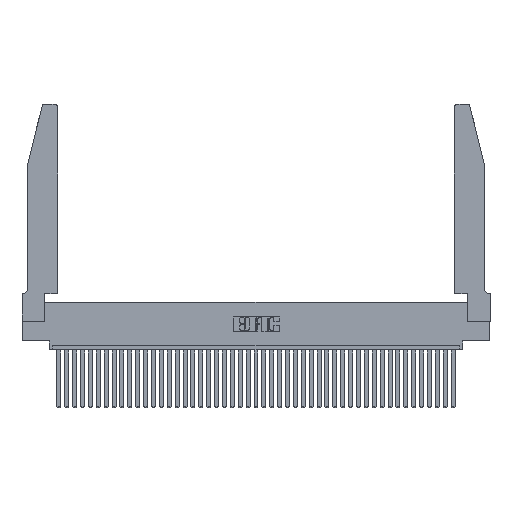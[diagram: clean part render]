
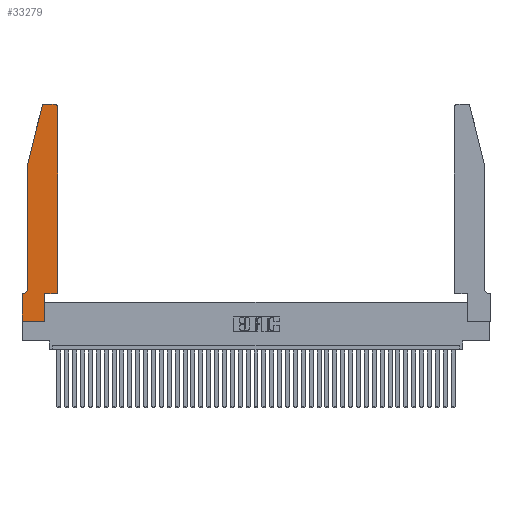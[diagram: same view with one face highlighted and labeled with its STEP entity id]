
A CAD part, top view. The second image highlights one B-rep face of the part: STEP entity #33279.
In plain terms, the highlighted planar face has unit normal (0, 0, 1).
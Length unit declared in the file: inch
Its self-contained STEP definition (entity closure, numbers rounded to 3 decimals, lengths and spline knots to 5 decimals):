
#1455 = CARTESIAN_POINT ( 'NONE',  ( 0., 0., 0.37 ) ) ;
#1532 = VECTOR ( 'NONE', #4703, 39.37008 ) ;
#1600 = DIRECTION ( 'NONE',  ( 0., 0., 1. ) ) ;
#2102 = EDGE_LOOP ( 'NONE', ( #39607, #27556, #12529, #35058, #14819, #30867, #3938, #31750, #32118, #39137, #9806, #36656 ) ) ;
#2121 = VERTEX_POINT ( 'NONE', #36961 ) ;
#2141 = CARTESIAN_POINT ( 'NONE',  ( 0.4205, 2.75, 0.37 ) ) ;
#2485 = VERTEX_POINT ( 'NONE', #36831 ) ;
#3154 = LINE ( 'NONE', #30062, #37539 ) ;
#3652 = CARTESIAN_POINT ( 'NONE',  ( 0., 0.35, 0.37 ) ) ;
#3937 = CIRCLE ( 'NONE', #37982, 0.03 ) ;
#3938 = ORIENTED_EDGE ( 'NONE', *, *, #39752, .T. ) ;
#4184 = LINE ( 'NONE', #41840, #13765 ) ;
#4213 = EDGE_CURVE ( 'NONE', #27043, #18013, #21855, .T. ) ;
#4671 = EDGE_CURVE ( 'NONE', #18013, #10865, #3154, .T. ) ;
#4703 = DIRECTION ( 'NONE',  ( 0., -1., 0. ) ) ;
#4770 = DIRECTION ( 'NONE',  ( 0., -1., 0. ) ) ;
#5153 = VERTEX_POINT ( 'NONE', #20958 ) ;
#6233 = VERTEX_POINT ( 'NONE', #3652 ) ;
#6235 = VECTOR ( 'NONE', #11917, 39.37008 ) ;
#6314 = CARTESIAN_POINT ( 'NONE',  ( 0.0755, 0.35, 0.37 ) ) ;
#7148 = EDGE_CURVE ( 'NONE', #34608, #27043, #18597, .T. ) ;
#7375 = VECTOR ( 'NONE', #31268, 39.37008 ) ;
#8874 = VECTOR ( 'NONE', #19285, 39.37008 ) ;
#8902 = EDGE_CURVE ( 'NONE', #31898, #6233, #24547, .T. ) ;
#9806 = ORIENTED_EDGE ( 'NONE', *, *, #24283, .T. ) ;
#10533 = EDGE_CURVE ( 'NONE', #2485, #30941, #40522, .T. ) ;
#10865 = VERTEX_POINT ( 'NONE', #31707 ) ;
#11106 = CARTESIAN_POINT ( 'NONE',  ( 0.284, 2.75, 0.37 ) ) ;
#11202 = DIRECTION ( 'NONE',  ( 1., 0., 0. ) ) ;
#11733 = CARTESIAN_POINT ( 'NONE',  ( 0.0055, 0.42, 0.37 ) ) ;
#11917 = DIRECTION ( 'NONE',  ( -0.239, -0.971, 0. ) ) ;
#12143 = AXIS2_PLACEMENT_3D ( 'NONE', #37515, #18132, #11202 ) ;
#12529 = ORIENTED_EDGE ( 'NONE', *, *, #4213, .T. ) ;
#12607 = VERTEX_POINT ( 'NONE', #2141 ) ;
#13274 = CARTESIAN_POINT ( 'NONE',  ( 0.4505, 0.35, 0.37 ) ) ;
#13550 = LINE ( 'NONE', #20067, #39370 ) ;
#13765 = VECTOR ( 'NONE', #19507, 39.37008 ) ;
#14819 = ORIENTED_EDGE ( 'NONE', *, *, #23988, .T. ) ;
#15023 = DIRECTION ( 'NONE',  ( 0., 0., -1. ) ) ;
#18013 = VERTEX_POINT ( 'NONE', #35134 ) ;
#18132 = DIRECTION ( 'NONE',  ( 0., 0., 1. ) ) ;
#18597 = CIRCLE ( 'NONE', #27298, 0.03 ) ;
#19285 = DIRECTION ( 'NONE',  ( -1., 0., 0. ) ) ;
#19507 = DIRECTION ( 'NONE',  ( 0., 1., 0. ) ) ;
#19769 = DIRECTION ( 'NONE',  ( 0., 1., 0. ) ) ;
#20067 = CARTESIAN_POINT ( 'NONE',  ( 0.2605, 2.75, 0.37 ) ) ;
#20542 = EDGE_CURVE ( 'NONE', #2121, #2485, #38345, .T. ) ;
#20958 = CARTESIAN_POINT ( 'NONE',  ( 0.4505, 2.72, 0.37 ) ) ;
#21148 = DIRECTION ( 'NONE',  ( 0., 0., 1. ) ) ;
#21514 = DIRECTION ( 'NONE',  ( -1., 0., 0. ) ) ;
#21816 = CARTESIAN_POINT ( 'NONE',  ( 0.0755, 2., 0.37 ) ) ;
#21855 = LINE ( 'NONE', #21816, #6235 ) ;
#22780 = CARTESIAN_POINT ( 'NONE',  ( 0.2865, 0.35, 0.37 ) ) ;
#23559 = AXIS2_PLACEMENT_3D ( 'NONE', #11733, #15023, #21514 ) ;
#23988 = EDGE_CURVE ( 'NONE', #10865, #31898, #40103, .T. ) ;
#24283 = EDGE_CURVE ( 'NONE', #30941, #5153, #4184, .T. ) ;
#24480 = FACE_OUTER_BOUND ( 'NONE', #2102, .T. ) ;
#24547 = LINE ( 'NONE', #6314, #8874 ) ;
#24636 = CARTESIAN_POINT ( 'NONE',  ( 0., 0., 0.37 ) ) ;
#25281 = CARTESIAN_POINT ( 'NONE',  ( 0.4505, 0.35, 0.37 ) ) ;
#27026 = EDGE_CURVE ( 'NONE', #12607, #34608, #13550, .T. ) ;
#27043 = VERTEX_POINT ( 'NONE', #30550 ) ;
#27231 = VECTOR ( 'NONE', #19769, 39.37008 ) ;
#27298 = AXIS2_PLACEMENT_3D ( 'NONE', #40869, #1600, #37095 ) ;
#27556 = ORIENTED_EDGE ( 'NONE', *, *, #7148, .T. ) ;
#27663 = DIRECTION ( 'NONE',  ( 1., 0., 0. ) ) ;
#27769 = EDGE_CURVE ( 'NONE', #5153, #12607, #3937, .T. ) ;
#28352 = LINE ( 'NONE', #1455, #1532 ) ;
#28815 = EDGE_CURVE ( 'NONE', #38876, #2121, #33159, .T. ) ;
#30062 = CARTESIAN_POINT ( 'NONE',  ( 0.0755, 2., 0.37 ) ) ;
#30550 = CARTESIAN_POINT ( 'NONE',  ( 0.25487, 2.72718, 0.37 ) ) ;
#30867 = ORIENTED_EDGE ( 'NONE', *, *, #8902, .T. ) ;
#30941 = VERTEX_POINT ( 'NONE', #25281 ) ;
#31268 = DIRECTION ( 'NONE',  ( 1., 0., 0. ) ) ;
#31707 = CARTESIAN_POINT ( 'NONE',  ( 0.0755, 0.42, 0.37 ) ) ;
#31750 = ORIENTED_EDGE ( 'NONE', *, *, #28815, .T. ) ;
#31808 = CARTESIAN_POINT ( 'NONE',  ( 0., 0., 0.37 ) ) ;
#31898 = VERTEX_POINT ( 'NONE', #36922 ) ;
#32118 = ORIENTED_EDGE ( 'NONE', *, *, #20542, .T. ) ;
#33159 = LINE ( 'NONE', #24636, #7375 ) ;
#33279 = ADVANCED_FACE ( 'NONE', ( #24480 ), #37104, .T. ) ;
#34608 = VERTEX_POINT ( 'NONE', #11106 ) ;
#35058 = ORIENTED_EDGE ( 'NONE', *, *, #4671, .T. ) ;
#35134 = CARTESIAN_POINT ( 'NONE',  ( 0.0755, 2., 0.37 ) ) ;
#35911 = DIRECTION ( 'NONE',  ( 1., 0., 0. ) ) ;
#36656 = ORIENTED_EDGE ( 'NONE', *, *, #27769, .T. ) ;
#36777 = DIRECTION ( 'NONE',  ( -1., 0., 0. ) ) ;
#36831 = CARTESIAN_POINT ( 'NONE',  ( 0.2865, 0.35, 0.37 ) ) ;
#36922 = CARTESIAN_POINT ( 'NONE',  ( 0.0055, 0.35, 0.37 ) ) ;
#36961 = CARTESIAN_POINT ( 'NONE',  ( 0.2865, 0., 0.37 ) ) ;
#37095 = DIRECTION ( 'NONE',  ( 1., 0., 0. ) ) ;
#37104 = PLANE ( 'NONE',  #12143 ) ;
#37515 = CARTESIAN_POINT ( 'NONE',  ( 0., 0.35, 0.37 ) ) ;
#37539 = VECTOR ( 'NONE', #4770, 39.37008 ) ;
#37982 = AXIS2_PLACEMENT_3D ( 'NONE', #41380, #21148, #27663 ) ;
#38345 = LINE ( 'NONE', #22780, #27231 ) ;
#38876 = VERTEX_POINT ( 'NONE', #31808 ) ;
#39043 = VECTOR ( 'NONE', #35911, 39.37008 ) ;
#39137 = ORIENTED_EDGE ( 'NONE', *, *, #10533, .T. ) ;
#39370 = VECTOR ( 'NONE', #36777, 39.37008 ) ;
#39607 = ORIENTED_EDGE ( 'NONE', *, *, #27026, .T. ) ;
#39752 = EDGE_CURVE ( 'NONE', #6233, #38876, #28352, .T. ) ;
#40103 = CIRCLE ( 'NONE', #23559, 0.07 ) ;
#40522 = LINE ( 'NONE', #13274, #39043 ) ;
#40869 = CARTESIAN_POINT ( 'NONE',  ( 0.284, 2.72, 0.37 ) ) ;
#41380 = CARTESIAN_POINT ( 'NONE',  ( 0.4205, 2.72, 0.37 ) ) ;
#41840 = CARTESIAN_POINT ( 'NONE',  ( 0.4505, 0.35, 0.37 ) ) ;
